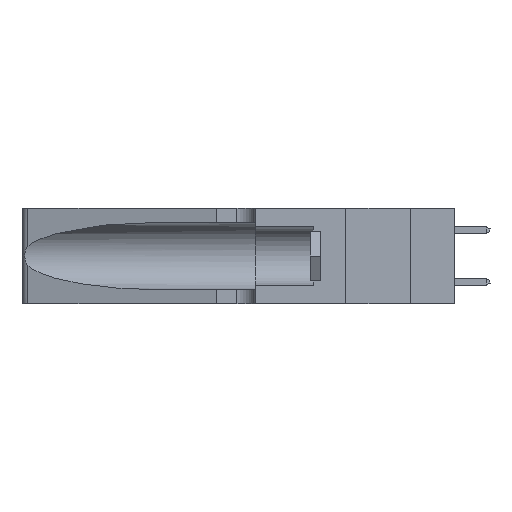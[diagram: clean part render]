
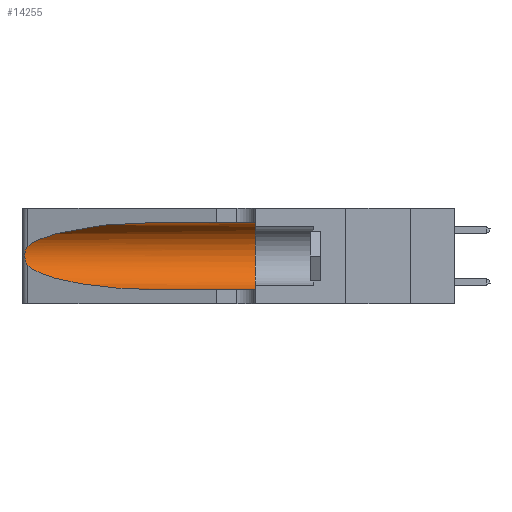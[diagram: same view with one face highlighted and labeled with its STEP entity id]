
A CAD part, left-side view. The second image highlights one B-rep face of the part: STEP entity #14255.
In plain terms, the highlighted cylindrical face has radius 3.308 mm (diameter 6.617 mm), a partial arc.
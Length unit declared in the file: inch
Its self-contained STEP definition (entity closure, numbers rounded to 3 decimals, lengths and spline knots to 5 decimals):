
#2038 = LINE ( 'NONE', #19762, #21413 ) ;
#2180 = CARTESIAN_POINT ( 'NONE',  ( 0.26017, 1.23833, 0.17102 ) ) ;
#2793 = CARTESIAN_POINT ( 'NONE',  ( 0.1305, 0.35, 0.31525 ) ) ;
#2896 = CARTESIAN_POINT ( 'NONE',  ( 0.2373, 1.15595, 0.28018 ) ) ;
#3765 = VERTEX_POINT ( 'NONE', #12509 ) ;
#3872 = EDGE_CURVE ( 'NONE', #10013, #7380, #31405, .T. ) ;
#4556 = VECTOR ( 'NONE', #25338, 39.37008 ) ;
#4710 = CARTESIAN_POINT ( 'NONE',  ( 0.25789, 1.23486, 0.15765 ) ) ;
#4883 = EDGE_CURVE ( 'NONE', #23563, #15651, #25582, .T. ) ;
#5572 = EDGE_CURVE ( 'NONE', #15651, #3765, #31403, .T. ) ;
#5616 = VERTEX_POINT ( 'NONE', #2793 ) ;
#5809 = DIRECTION ( 'NONE',  ( 0., 1., 0. ) ) ;
#5988 = CARTESIAN_POINT ( 'NONE',  ( 0.1305, 1.61858, 0.185 ) ) ;
#7160 = ORIENTED_EDGE ( 'NONE', *, *, #5572, .T. ) ;
#7255 = CARTESIAN_POINT ( 'NONE',  ( 0.25555, 1.22993, 0.14849 ) ) ;
#7380 = VERTEX_POINT ( 'NONE', #27078 ) ;
#8210 = FACE_OUTER_BOUND ( 'NONE', #10136, .T. ) ;
#10013 = VERTEX_POINT ( 'NONE', #21018 ) ;
#10136 = EDGE_LOOP ( 'NONE', ( #21850, #22605, #17056, #7160, #23356, #24541 ) ) ;
#11379 = B_SPLINE_CURVE_WITH_KNOTS ( 'NONE', 3,
 ( #24825, #29776, #27366, #12222, #29883, #14764, #32391, #17310, #2180, #19862, #4710, #22385, #7255, #24933 ),
 .UNSPECIFIED., .F., .F.,
 ( 4, 2, 2, 2, 2, 2, 4 ),
 ( 0., 0.00027, 0.00053, 0.00107, 0.0016, 0.00187, 0.00214 ),
 .UNSPECIFIED. ) ;
#12222 = CARTESIAN_POINT ( 'NONE',  ( 0.25787, 1.23484, 0.2124 ) ) ;
#12509 = CARTESIAN_POINT ( 'NONE',  ( 0.1305, 0.35, 0.05475 ) ) ;
#12639 = EDGE_CURVE ( 'NONE', #5616, #3765, #15433, .T. ) ;
#14255 = ADVANCED_FACE ( 'NONE', ( #8210 ), #20880, .F. ) ;
#14526 = CARTESIAN_POINT ( 'NONE',  ( 0.2373, 1.15595, 0.08982 ) ) ;
#14764 = CARTESIAN_POINT ( 'NONE',  ( 0.26018, 1.23835, 0.19895 ) ) ;
#15433 = CIRCLE ( 'NONE', #24082, 0.13025 ) ;
#15651 = VERTEX_POINT ( 'NONE', #28761 ) ;
#16057 = DIRECTION ( 'NONE',  ( 0., -1., 0. ) ) ;
#16951 = CARTESIAN_POINT ( 'NONE',  ( 0.25487, 1.22718, 0.14631 ) ) ;
#17056 = ORIENTED_EDGE ( 'NONE', *, *, #4883, .T. ) ;
#17069 = CARTESIAN_POINT ( 'NONE',  ( 0.25487, 1.22718, 0.14631 ) ) ;
#17310 = CARTESIAN_POINT ( 'NONE',  ( 0.26075, 1.23896, 0.178 ) ) ;
#17708 = CARTESIAN_POINT ( 'NONE',  ( 0.1305, 1.61858, 0.05475 ) ) ;
#19629 = CARTESIAN_POINT ( 'NONE',  ( 0.1305, 0.72297, 0.05475 ) ) ;
#19762 = CARTESIAN_POINT ( 'NONE',  ( 0.1305, 1.61858, 0.31525 ) ) ;
#19862 = CARTESIAN_POINT ( 'NONE',  ( 0.25856, 1.23593, 0.16098 ) ) ;
#20880 = CYLINDRICAL_SURFACE ( 'NONE', #24345, 0.13025 ) ;
#20982 = CARTESIAN_POINT ( 'NONE',  ( 0.1305, 0.35, 0.185 ) ) ;
#21018 = CARTESIAN_POINT ( 'NONE',  ( 0.1305, 0.72297, 0.31525 ) ) ;
#21413 = VECTOR ( 'NONE', #22284, 39.37008 ) ;
#21850 = ORIENTED_EDGE ( 'NONE', *, *, #3872, .T. ) ;
#22284 = DIRECTION ( 'NONE',  ( 0., -1., 0. ) ) ;
#22385 = CARTESIAN_POINT ( 'NONE',  ( 0.25639, 1.23186, 0.15144 ) ) ;
#22605 = ORIENTED_EDGE ( 'NONE', *, *, #29272, .T. ) ;
#23356 = ORIENTED_EDGE ( 'NONE', *, *, #12639, .F. ) ;
#23486 = DIRECTION ( 'NONE',  ( 0., 0., 1. ) ) ;
#23563 = VERTEX_POINT ( 'NONE', #16951 ) ;
#24082 = AXIS2_PLACEMENT_3D ( 'NONE', #20982, #5809, #23486 ) ;
#24345 = AXIS2_PLACEMENT_3D ( 'NONE', #5988, #16057, #31152 ) ;
#24541 = ORIENTED_EDGE ( 'NONE', *, *, #31149, .F. ) ;
#24825 = CARTESIAN_POINT ( 'NONE',  ( 0.25487, 1.22718, 0.22369 ) ) ;
#24933 = CARTESIAN_POINT ( 'NONE',  ( 0.25487, 1.22718, 0.14631 ) ) ;
#25338 = DIRECTION ( 'NONE',  ( 0., -1., 0. ) ) ;
#25582 =( BOUNDED_CURVE ( )  B_SPLINE_CURVE ( 3, ( #17069, #14526, #27138, #19629 ),
 .UNSPECIFIED., .F., .T. ) 
 B_SPLINE_CURVE_WITH_KNOTS ( ( 4, 4 ),
 ( 3.44316, 4.71239 ),
 .UNSPECIFIED. ) 
 CURVE ( )  GEOMETRIC_REPRESENTATION_ITEM ( )  RATIONAL_B_SPLINE_CURVE ( ( 1., 0.87, 0.87, 1. ) ) 
 REPRESENTATION_ITEM ( '' )  );
#25665 = CARTESIAN_POINT ( 'NONE',  ( 0.18966, 0.96281, 0.31525 ) ) ;
#27078 = CARTESIAN_POINT ( 'NONE',  ( 0.25487, 1.22718, 0.22369 ) ) ;
#27138 = CARTESIAN_POINT ( 'NONE',  ( 0.18966, 0.96281, 0.05475 ) ) ;
#27366 = CARTESIAN_POINT ( 'NONE',  ( 0.25639, 1.23184, 0.21858 ) ) ;
#28181 = CARTESIAN_POINT ( 'NONE',  ( 0.1305, 0.72297, 0.31525 ) ) ;
#28761 = CARTESIAN_POINT ( 'NONE',  ( 0.1305, 0.72297, 0.05475 ) ) ;
#29272 = EDGE_CURVE ( 'NONE', #7380, #23563, #11379, .T. ) ;
#29776 = CARTESIAN_POINT ( 'NONE',  ( 0.25555, 1.22994, 0.2215 ) ) ;
#29883 = CARTESIAN_POINT ( 'NONE',  ( 0.25854, 1.2359, 0.20912 ) ) ;
#30699 = CARTESIAN_POINT ( 'NONE',  ( 0.25487, 1.22718, 0.22369 ) ) ;
#31149 = EDGE_CURVE ( 'NONE', #10013, #5616, #2038, .T. ) ;
#31152 = DIRECTION ( 'NONE',  ( 0., 0., -1. ) ) ;
#31403 = LINE ( 'NONE', #17708, #4556 ) ;
#31405 =( BOUNDED_CURVE ( )  B_SPLINE_CURVE ( 3, ( #28181, #25665, #2896, #30699 ),
 .UNSPECIFIED., .F., .T. ) 
 B_SPLINE_CURVE_WITH_KNOTS ( ( 4, 4 ),
 ( 1.5708, 2.84003 ),
 .UNSPECIFIED. ) 
 CURVE ( )  GEOMETRIC_REPRESENTATION_ITEM ( )  RATIONAL_B_SPLINE_CURVE ( ( 1., 0.87, 0.87, 1. ) ) 
 REPRESENTATION_ITEM ( '' )  );
#32391 = CARTESIAN_POINT ( 'NONE',  ( 0.26075, 1.23896, 0.19203 ) ) ;
